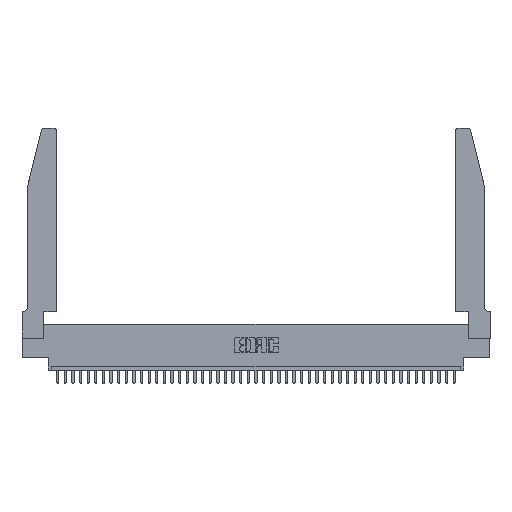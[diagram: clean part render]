
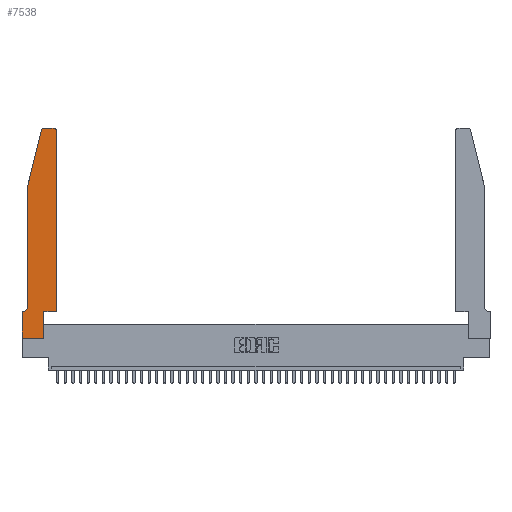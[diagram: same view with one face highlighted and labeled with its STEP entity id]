
A CAD part, top view. The second image highlights one B-rep face of the part: STEP entity #7538.
In plain terms, the highlighted planar face has unit normal (0, 0, 1).
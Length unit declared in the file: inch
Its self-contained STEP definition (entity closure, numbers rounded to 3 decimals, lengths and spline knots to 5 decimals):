
#45 = VERTEX_POINT ( 'NONE', #5617 ) ;
#78 = CARTESIAN_POINT ( 'NONE',  ( 0.25487, 2.72718, 0.37 ) ) ;
#1028 = CARTESIAN_POINT ( 'NONE',  ( 0.0055, 0.42, 0.37 ) ) ;
#1224 = ORIENTED_EDGE ( 'NONE', *, *, #18398, .T. ) ;
#1279 = LINE ( 'NONE', #33706, #40100 ) ;
#1442 = DIRECTION ( 'NONE',  ( 1., 0., 0. ) ) ;
#2191 = ORIENTED_EDGE ( 'NONE', *, *, #29775, .T. ) ;
#2277 = ORIENTED_EDGE ( 'NONE', *, *, #18245, .T. ) ;
#2605 = CARTESIAN_POINT ( 'NONE',  ( 0.4205, 2.72, 0.37 ) ) ;
#3429 = EDGE_CURVE ( 'NONE', #6471, #4085, #17972, .T. ) ;
#3920 = EDGE_CURVE ( 'NONE', #20471, #5553, #9035, .T. ) ;
#4071 = VECTOR ( 'NONE', #29044, 39.37008 ) ;
#4085 = VERTEX_POINT ( 'NONE', #19353 ) ;
#4872 = CARTESIAN_POINT ( 'NONE',  ( 0.4205, 2.75, 0.37 ) ) ;
#5553 = VERTEX_POINT ( 'NONE', #8033 ) ;
#5617 = CARTESIAN_POINT ( 'NONE',  ( 0.0755, 2., 0.37 ) ) ;
#5971 = DIRECTION ( 'NONE',  ( 0., 0., 1. ) ) ;
#6387 = CARTESIAN_POINT ( 'NONE',  ( 0.4505, 0.35, 0.37 ) ) ;
#6471 = VERTEX_POINT ( 'NONE', #14935 ) ;
#7003 = CARTESIAN_POINT ( 'NONE',  ( 0.4505, 0.35, 0.37 ) ) ;
#7017 = CARTESIAN_POINT ( 'NONE',  ( 0., 0.35, 0.37 ) ) ;
#7153 = CARTESIAN_POINT ( 'NONE',  ( 0.2865, 0.35, 0.37 ) ) ;
#7384 = ORIENTED_EDGE ( 'NONE', *, *, #3920, .T. ) ;
#7538 = ADVANCED_FACE ( 'NONE', ( #40306 ), #23037, .T. ) ;
#7999 = CIRCLE ( 'NONE', #19639, 0.03 ) ;
#8027 = DIRECTION ( 'NONE',  ( 0., 0., 1. ) ) ;
#8033 = CARTESIAN_POINT ( 'NONE',  ( 0.284, 2.75, 0.37 ) ) ;
#8548 = VECTOR ( 'NONE', #31345, 39.37008 ) ;
#8899 = AXIS2_PLACEMENT_3D ( 'NONE', #1028, #24495, #27871 ) ;
#9035 = LINE ( 'NONE', #16361, #24731 ) ;
#9383 = DIRECTION ( 'NONE',  ( 0., 0., 1. ) ) ;
#9593 = LINE ( 'NONE', #7003, #25372 ) ;
#9784 = DIRECTION ( 'NONE',  ( -1., 0., 0. ) ) ;
#9825 = CARTESIAN_POINT ( 'NONE',  ( 0., 0.35, 0.37 ) ) ;
#9912 = LINE ( 'NONE', #36087, #17717 ) ;
#10935 = CARTESIAN_POINT ( 'NONE',  ( 0.4505, 2.72, 0.37 ) ) ;
#11532 = ORIENTED_EDGE ( 'NONE', *, *, #26013, .T. ) ;
#12337 = LINE ( 'NONE', #18268, #28018 ) ;
#14665 = CARTESIAN_POINT ( 'NONE',  ( 0.0755, 0.35, 0.37 ) ) ;
#14935 = CARTESIAN_POINT ( 'NONE',  ( 0., 0., 0.37 ) ) ;
#16361 = CARTESIAN_POINT ( 'NONE',  ( 0.2605, 2.75, 0.37 ) ) ;
#17221 = DIRECTION ( 'NONE',  ( 0., 1., 0. ) ) ;
#17539 = VECTOR ( 'NONE', #17221, 39.37008 ) ;
#17717 = VECTOR ( 'NONE', #39473, 39.37008 ) ;
#17972 = LINE ( 'NONE', #34664, #27380 ) ;
#18245 = EDGE_CURVE ( 'NONE', #20255, #30297, #9593, .T. ) ;
#18248 = CARTESIAN_POINT ( 'NONE',  ( 0.284, 2.72, 0.37 ) ) ;
#18268 = CARTESIAN_POINT ( 'NONE',  ( 0.0755, 2., 0.37 ) ) ;
#18398 = EDGE_CURVE ( 'NONE', #30297, #20471, #7999, .T. ) ;
#18601 = ORIENTED_EDGE ( 'NONE', *, *, #3429, .T. ) ;
#19353 = CARTESIAN_POINT ( 'NONE',  ( 0.2865, 0., 0.37 ) ) ;
#19639 = AXIS2_PLACEMENT_3D ( 'NONE', #2605, #5971, #32444 ) ;
#19864 = ORIENTED_EDGE ( 'NONE', *, *, #28879, .T. ) ;
#20255 = VERTEX_POINT ( 'NONE', #6387 ) ;
#20336 = ORIENTED_EDGE ( 'NONE', *, *, #39409, .T. ) ;
#20471 = VERTEX_POINT ( 'NONE', #4872 ) ;
#21515 = DIRECTION ( 'NONE',  ( -0.239, -0.971, 0. ) ) ;
#21545 = ORIENTED_EDGE ( 'NONE', *, *, #43421, .T. ) ;
#22745 = LINE ( 'NONE', #14665, #8548 ) ;
#23037 = PLANE ( 'NONE',  #24464 ) ;
#23316 = DIRECTION ( 'NONE',  ( 1., 0., 0. ) ) ;
#23488 = EDGE_CURVE ( 'NONE', #45, #33168, #39715, .T. ) ;
#23631 = DIRECTION ( 'NONE',  ( 0., -1., 0. ) ) ;
#24442 = ORIENTED_EDGE ( 'NONE', *, *, #23488, .T. ) ;
#24464 = AXIS2_PLACEMENT_3D ( 'NONE', #9825, #9383, #23316 ) ;
#24495 = DIRECTION ( 'NONE',  ( 0., 0., -1. ) ) ;
#24731 = VECTOR ( 'NONE', #9784, 39.37008 ) ;
#25372 = VECTOR ( 'NONE', #39810, 39.37008 ) ;
#25508 = LINE ( 'NONE', #32947, #17539 ) ;
#26013 = EDGE_CURVE ( 'NONE', #4085, #29244, #25508, .T. ) ;
#26129 = VERTEX_POINT ( 'NONE', #33251 ) ;
#26646 = CARTESIAN_POINT ( 'NONE',  ( 0.0755, 0.42, 0.37 ) ) ;
#27380 = VECTOR ( 'NONE', #1442, 39.37008 ) ;
#27871 = DIRECTION ( 'NONE',  ( -1., 0., 0. ) ) ;
#28018 = VECTOR ( 'NONE', #21515, 39.37008 ) ;
#28449 = CARTESIAN_POINT ( 'NONE',  ( 0.0755, 2., 0.37 ) ) ;
#28879 = EDGE_CURVE ( 'NONE', #5553, #40518, #30436, .T. ) ;
#29044 = DIRECTION ( 'NONE',  ( 0., -1., 0. ) ) ;
#29079 = VERTEX_POINT ( 'NONE', #7017 ) ;
#29244 = VERTEX_POINT ( 'NONE', #7153 ) ;
#29775 = EDGE_CURVE ( 'NONE', #29079, #6471, #1279, .T. ) ;
#30297 = VERTEX_POINT ( 'NONE', #10935 ) ;
#30436 = CIRCLE ( 'NONE', #36329, 0.03 ) ;
#31345 = DIRECTION ( 'NONE',  ( -1., 0., 0. ) ) ;
#32444 = DIRECTION ( 'NONE',  ( 1., 0., 0. ) ) ;
#32462 = ORIENTED_EDGE ( 'NONE', *, *, #41303, .T. ) ;
#32716 = EDGE_LOOP ( 'NONE', ( #7384, #19864, #21545, #24442, #32462, #20336, #2191, #18601, #11532, #38887, #2277, #1224 ) ) ;
#32947 = CARTESIAN_POINT ( 'NONE',  ( 0.2865, 0.35, 0.37 ) ) ;
#33168 = VERTEX_POINT ( 'NONE', #26646 ) ;
#33251 = CARTESIAN_POINT ( 'NONE',  ( 0.0055, 0.35, 0.37 ) ) ;
#33706 = CARTESIAN_POINT ( 'NONE',  ( 0., 0., 0.37 ) ) ;
#34664 = CARTESIAN_POINT ( 'NONE',  ( 0., 0., 0.37 ) ) ;
#34794 = DIRECTION ( 'NONE',  ( 1., 0., 0. ) ) ;
#35417 = EDGE_CURVE ( 'NONE', #29244, #20255, #9912, .T. ) ;
#36087 = CARTESIAN_POINT ( 'NONE',  ( 0.4505, 0.35, 0.37 ) ) ;
#36329 = AXIS2_PLACEMENT_3D ( 'NONE', #18248, #8027, #34794 ) ;
#38887 = ORIENTED_EDGE ( 'NONE', *, *, #35417, .T. ) ;
#39409 = EDGE_CURVE ( 'NONE', #26129, #29079, #22745, .T. ) ;
#39473 = DIRECTION ( 'NONE',  ( 1., 0., 0. ) ) ;
#39715 = LINE ( 'NONE', #28449, #4071 ) ;
#39810 = DIRECTION ( 'NONE',  ( 0., 1., 0. ) ) ;
#40100 = VECTOR ( 'NONE', #23631, 39.37008 ) ;
#40306 = FACE_OUTER_BOUND ( 'NONE', #32716, .T. ) ;
#40518 = VERTEX_POINT ( 'NONE', #78 ) ;
#41291 = CIRCLE ( 'NONE', #8899, 0.07 ) ;
#41303 = EDGE_CURVE ( 'NONE', #33168, #26129, #41291, .T. ) ;
#43421 = EDGE_CURVE ( 'NONE', #40518, #45, #12337, .T. ) ;
